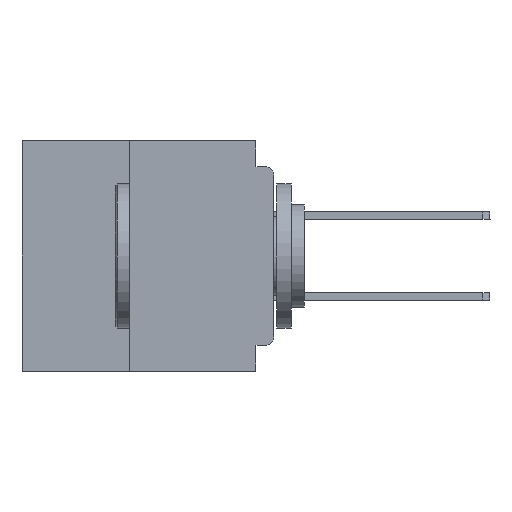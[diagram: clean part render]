
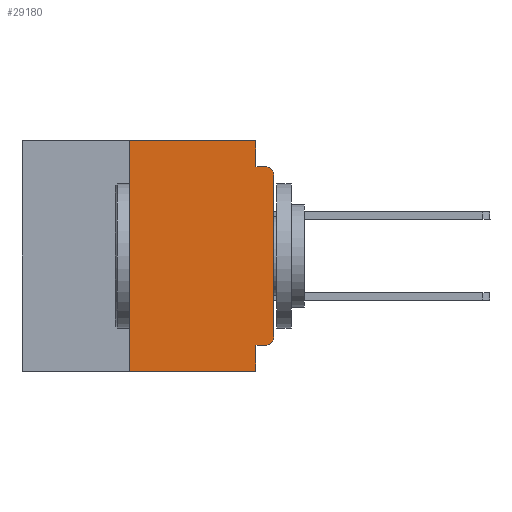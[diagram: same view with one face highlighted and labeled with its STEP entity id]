
A CAD part, left-side view. The second image highlights one B-rep face of the part: STEP entity #29180.
In plain terms, the highlighted planar face has unit normal (-1, 0, 0).
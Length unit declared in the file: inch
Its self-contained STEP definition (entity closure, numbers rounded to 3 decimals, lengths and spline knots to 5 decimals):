
#981 = PLANE ( 'NONE',  #50223 ) ;
#1204 = LINE ( 'NONE', #40493, #52206 ) ;
#1530 = VECTOR ( 'NONE', #57466, 39.37008 ) ;
#2034 = DIRECTION ( 'NONE',  ( -1., 0., 0. ) ) ;
#3135 = LINE ( 'NONE', #16840, #1530 ) ;
#3420 = FACE_OUTER_BOUND ( 'NONE', #22421, .T. ) ;
#5510 = EDGE_CURVE ( 'NONE', #62000, #47971, #55644, .T. ) ;
#5744 = LINE ( 'NONE', #19724, #31292 ) ;
#6110 = AXIS2_PLACEMENT_3D ( 'NONE', #44081, #13560, #49153 ) ;
#6899 = CARTESIAN_POINT ( 'NONE',  ( 0., 0.437, -0.4 ) ) ;
#8117 = VERTEX_POINT ( 'NONE', #42326 ) ;
#9196 = VERTEX_POINT ( 'NONE', #56906 ) ;
#10098 = EDGE_CURVE ( 'NONE', #47971, #8117, #5744, .T. ) ;
#10161 = DIRECTION ( 'NONE',  ( 0., -1., 0. ) ) ;
#11269 = EDGE_CURVE ( 'NONE', #33656, #33073, #17025, .T. ) ;
#11317 = DIRECTION ( 'NONE',  ( 0., 0., -1. ) ) ;
#12370 = VERTEX_POINT ( 'NONE', #46960 ) ;
#13305 = VERTEX_POINT ( 'NONE', #49469 ) ;
#13502 = VECTOR ( 'NONE', #37741, 39.37008 ) ;
#13540 = ORIENTED_EDGE ( 'NONE', *, *, #61190, .T. ) ;
#13560 = DIRECTION ( 'NONE',  ( -1., 0., 0. ) ) ;
#15427 = VECTOR ( 'NONE', #23355, 39.37008 ) ;
#15889 = ORIENTED_EDGE ( 'NONE', *, *, #18450, .F. ) ;
#16840 = CARTESIAN_POINT ( 'NONE',  ( 0., 0., 0. ) ) ;
#17025 = LINE ( 'NONE', #48758, #15427 ) ;
#18450 = EDGE_CURVE ( 'NONE', #12370, #33656, #1204, .T. ) ;
#18702 = EDGE_CURVE ( 'NONE', #13305, #31114, #21154, .T. ) ;
#19724 = CARTESIAN_POINT ( 'NONE',  ( 0., 0.031, -0.4 ) ) ;
#21154 = CIRCLE ( 'NONE', #59598, 0.015 ) ;
#21210 = ORIENTED_EDGE ( 'NONE', *, *, #38855, .F. ) ;
#22421 = EDGE_LOOP ( 'NONE', ( #13540, #25131, #62382, #63535, #15889, #21210, #32416, #39614, #51570, #57614 ) ) ;
#22539 = CARTESIAN_POINT ( 'NONE',  ( 0., 0.015, -0.355 ) ) ;
#23355 = DIRECTION ( 'NONE',  ( 0., 0., -1. ) ) ;
#23869 = VECTOR ( 'NONE', #49429, 39.37008 ) ;
#25131 = ORIENTED_EDGE ( 'NONE', *, *, #18702, .T. ) ;
#27409 = LINE ( 'NONE', #6899, #52856 ) ;
#29180 = ADVANCED_FACE ( 'NONE', ( #3420 ), #981, .F. ) ;
#31114 = VERTEX_POINT ( 'NONE', #62115 ) ;
#31292 = VECTOR ( 'NONE', #50180, 39.37008 ) ;
#32416 = ORIENTED_EDGE ( 'NONE', *, *, #44924, .T. ) ;
#32629 = CARTESIAN_POINT ( 'NONE',  ( 0., 0.015, -0.06 ) ) ;
#33073 = VERTEX_POINT ( 'NONE', #56380 ) ;
#33656 = VERTEX_POINT ( 'NONE', #40673 ) ;
#37487 = LINE ( 'NONE', #64446, #23869 ) ;
#37741 = DIRECTION ( 'NONE',  ( 0., 1., 0. ) ) ;
#37792 = DIRECTION ( 'NONE',  ( 0., 0., -1. ) ) ;
#38855 = EDGE_CURVE ( 'NONE', #9196, #12370, #37487, .T. ) ;
#39614 = ORIENTED_EDGE ( 'NONE', *, *, #10098, .F. ) ;
#40493 = CARTESIAN_POINT ( 'NONE',  ( 0., 0.437, 0. ) ) ;
#40673 = CARTESIAN_POINT ( 'NONE',  ( 0., 0.031, 0. ) ) ;
#41870 = DIRECTION ( 'NONE',  ( 1., 0., 0. ) ) ;
#42326 = CARTESIAN_POINT ( 'NONE',  ( 0., 0.031, -0.4 ) ) ;
#42629 = DIRECTION ( 'NONE',  ( 0., -1., 0. ) ) ;
#44081 = CARTESIAN_POINT ( 'NONE',  ( 0., 0.015, -0.34 ) ) ;
#44924 = EDGE_CURVE ( 'NONE', #9196, #8117, #27409, .T. ) ;
#45975 = CARTESIAN_POINT ( 'NONE',  ( 0., 0.031, -0.355 ) ) ;
#46960 = CARTESIAN_POINT ( 'NONE',  ( 0., 0.25, 0. ) ) ;
#47971 = VERTEX_POINT ( 'NONE', #45975 ) ;
#48758 = CARTESIAN_POINT ( 'NONE',  ( 0., 0.031, 0. ) ) ;
#49153 = DIRECTION ( 'NONE',  ( 0., 0., -1. ) ) ;
#49429 = DIRECTION ( 'NONE',  ( 0., 0., 1. ) ) ;
#49469 = CARTESIAN_POINT ( 'NONE',  ( 0., 0., -0.06 ) ) ;
#50180 = DIRECTION ( 'NONE',  ( 0., 0., -1. ) ) ;
#50223 = AXIS2_PLACEMENT_3D ( 'NONE', #61919, #41870, #11317 ) ;
#51094 = CARTESIAN_POINT ( 'NONE',  ( 0., 0., -0.34 ) ) ;
#51218 = CARTESIAN_POINT ( 'NONE',  ( 0., 0., -0.045 ) ) ;
#51570 = ORIENTED_EDGE ( 'NONE', *, *, #5510, .F. ) ;
#52206 = VECTOR ( 'NONE', #10161, 39.37008 ) ;
#52856 = VECTOR ( 'NONE', #42629, 39.37008 ) ;
#53027 = VECTOR ( 'NONE', #61135, 39.37008 ) ;
#54176 = CIRCLE ( 'NONE', #6110, 0.015 ) ;
#54608 = LINE ( 'NONE', #51218, #53027 ) ;
#54706 = EDGE_CURVE ( 'NONE', #33073, #31114, #54608, .T. ) ;
#55644 = LINE ( 'NONE', #62908, #13502 ) ;
#56380 = CARTESIAN_POINT ( 'NONE',  ( 0., 0.031, -0.045 ) ) ;
#56906 = CARTESIAN_POINT ( 'NONE',  ( 0., 0.25, -0.4 ) ) ;
#57466 = DIRECTION ( 'NONE',  ( 0., 0., 1. ) ) ;
#57614 = ORIENTED_EDGE ( 'NONE', *, *, #60785, .T. ) ;
#59598 = AXIS2_PLACEMENT_3D ( 'NONE', #32629, #2034, #37792 ) ;
#60785 = EDGE_CURVE ( 'NONE', #62000, #63079, #54176, .T. ) ;
#61135 = DIRECTION ( 'NONE',  ( 0., -1., 0. ) ) ;
#61190 = EDGE_CURVE ( 'NONE', #63079, #13305, #3135, .T. ) ;
#61919 = CARTESIAN_POINT ( 'NONE',  ( 0., 0.437, 0. ) ) ;
#62000 = VERTEX_POINT ( 'NONE', #22539 ) ;
#62115 = CARTESIAN_POINT ( 'NONE',  ( 0., 0.015, -0.045 ) ) ;
#62382 = ORIENTED_EDGE ( 'NONE', *, *, #54706, .F. ) ;
#62908 = CARTESIAN_POINT ( 'NONE',  ( 0., 0., -0.355 ) ) ;
#63079 = VERTEX_POINT ( 'NONE', #51094 ) ;
#63535 = ORIENTED_EDGE ( 'NONE', *, *, #11269, .F. ) ;
#64446 = CARTESIAN_POINT ( 'NONE',  ( 0., 0.25, -0.4 ) ) ;
